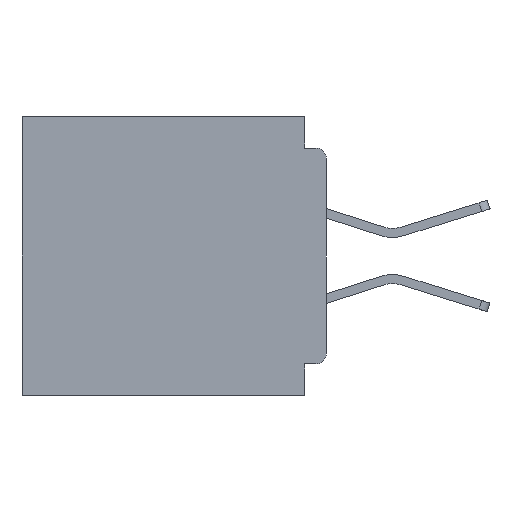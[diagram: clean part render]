
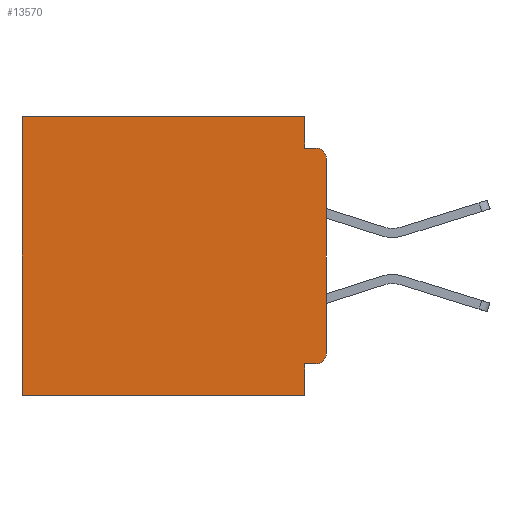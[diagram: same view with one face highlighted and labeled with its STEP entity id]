
A CAD part, left-side view. The second image highlights one B-rep face of the part: STEP entity #13570.
In plain terms, the highlighted planar face has unit normal (-1, 0, 0).
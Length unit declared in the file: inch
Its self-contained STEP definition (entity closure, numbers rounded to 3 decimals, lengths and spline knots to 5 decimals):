
#311 = EDGE_CURVE ( 'NONE', #14946, #16887, #39756, .T. ) ;
#653 = VECTOR ( 'NONE', #35557, 39.37008 ) ;
#1176 = VERTEX_POINT ( 'NONE', #3523 ) ;
#2168 = VERTEX_POINT ( 'NONE', #37568 ) ;
#3523 = CARTESIAN_POINT ( 'NONE',  ( 0.3, 0.031, -0.355 ) ) ;
#4334 = AXIS2_PLACEMENT_3D ( 'NONE', #11933, #9984, #10030 ) ;
#4850 = ORIENTED_EDGE ( 'NONE', *, *, #23393, .T. ) ;
#4950 = ORIENTED_EDGE ( 'NONE', *, *, #31621, .T. ) ;
#4956 = AXIS2_PLACEMENT_3D ( 'NONE', #25926, #29828, #6241 ) ;
#5565 = EDGE_CURVE ( 'NONE', #2168, #43491, #44742, .T. ) ;
#5735 = CARTESIAN_POINT ( 'NONE',  ( 0.3, 0.031, -0.045 ) ) ;
#6241 = DIRECTION ( 'NONE',  ( 0., 0., -1. ) ) ;
#8065 = CARTESIAN_POINT ( 'NONE',  ( 0.3, 0.437, -0.4 ) ) ;
#8159 = DIRECTION ( 'NONE',  ( 0., 0., -1. ) ) ;
#8387 = CARTESIAN_POINT ( 'NONE',  ( 0.3, 0., -0.34 ) ) ;
#9984 = DIRECTION ( 'NONE',  ( -1., 0., 0. ) ) ;
#10030 = DIRECTION ( 'NONE',  ( 0., 0., -1. ) ) ;
#10663 = ORIENTED_EDGE ( 'NONE', *, *, #46131, .F. ) ;
#10759 = DIRECTION ( 'NONE',  ( 0., 1., 0. ) ) ;
#11933 = CARTESIAN_POINT ( 'NONE',  ( 0.3, 0.015, -0.06 ) ) ;
#12539 = VECTOR ( 'NONE', #13088, 39.37008 ) ;
#13088 = DIRECTION ( 'NONE',  ( 0., 0., -1. ) ) ;
#13570 = ADVANCED_FACE ( 'NONE', ( #33282 ), #49184, .F. ) ;
#13924 = ORIENTED_EDGE ( 'NONE', *, *, #36365, .F. ) ;
#14374 = VERTEX_POINT ( 'NONE', #38635 ) ;
#14946 = VERTEX_POINT ( 'NONE', #18357 ) ;
#16887 = VERTEX_POINT ( 'NONE', #8387 ) ;
#17901 = LINE ( 'NONE', #8065, #653 ) ;
#18357 = CARTESIAN_POINT ( 'NONE',  ( 0.3, 0.015, -0.355 ) ) ;
#18718 = LINE ( 'NONE', #46426, #47393 ) ;
#19188 = LINE ( 'NONE', #28607, #38805 ) ;
#19637 = LINE ( 'NONE', #32131, #38030 ) ;
#20195 = LINE ( 'NONE', #35977, #46417 ) ;
#21438 = EDGE_CURVE ( 'NONE', #14946, #1176, #18718, .T. ) ;
#23393 = EDGE_CURVE ( 'NONE', #29288, #49319, #17901, .T. ) ;
#24069 = CARTESIAN_POINT ( 'NONE',  ( 0.3, 0.031, 0. ) ) ;
#24541 = VERTEX_POINT ( 'NONE', #5735 ) ;
#25926 = CARTESIAN_POINT ( 'NONE',  ( 0.3, 0., -0.4 ) ) ;
#26956 = ORIENTED_EDGE ( 'NONE', *, *, #5565, .T. ) ;
#27587 = CARTESIAN_POINT ( 'NONE',  ( 0.3, 0.437, -0.4 ) ) ;
#28607 = CARTESIAN_POINT ( 'NONE',  ( 0.3, 0., -0.045 ) ) ;
#29288 = VERTEX_POINT ( 'NONE', #43080 ) ;
#29828 = DIRECTION ( 'NONE',  ( 1., 0., 0. ) ) ;
#30958 = EDGE_CURVE ( 'NONE', #2168, #16887, #19637, .T. ) ;
#31077 = CARTESIAN_POINT ( 'NONE',  ( 0.3, 0.031, -0.4 ) ) ;
#31420 = EDGE_LOOP ( 'NONE', ( #39469, #26956, #32062, #37504, #4950, #4850, #13924, #10663, #32097, #32946 ) ) ;
#31621 = EDGE_CURVE ( 'NONE', #14374, #29288, #20195, .T. ) ;
#32062 = ORIENTED_EDGE ( 'NONE', *, *, #47541, .F. ) ;
#32097 = ORIENTED_EDGE ( 'NONE', *, *, #21438, .F. ) ;
#32131 = CARTESIAN_POINT ( 'NONE',  ( 0.3, 0., -0.4 ) ) ;
#32946 = ORIENTED_EDGE ( 'NONE', *, *, #311, .T. ) ;
#33282 = FACE_OUTER_BOUND ( 'NONE', #31420, .T. ) ;
#33768 = CARTESIAN_POINT ( 'NONE',  ( 0.3, 0.015, -0.045 ) ) ;
#34893 = DIRECTION ( 'NONE',  ( 0., 1., 0. ) ) ;
#35557 = DIRECTION ( 'NONE',  ( 0., 0., -1. ) ) ;
#35602 = VECTOR ( 'NONE', #8159, 39.37008 ) ;
#35977 = CARTESIAN_POINT ( 'NONE',  ( 0.3, 0., 0. ) ) ;
#36038 = DIRECTION ( 'NONE',  ( 0., 0., -1. ) ) ;
#36232 = VECTOR ( 'NONE', #10759, 39.37008 ) ;
#36365 = EDGE_CURVE ( 'NONE', #48609, #49319, #46570, .T. ) ;
#36580 = CARTESIAN_POINT ( 'NONE',  ( 0.3, 0.031, -0.4 ) ) ;
#36820 = LINE ( 'NONE', #24069, #35602 ) ;
#37504 = ORIENTED_EDGE ( 'NONE', *, *, #48725, .F. ) ;
#37568 = CARTESIAN_POINT ( 'NONE',  ( 0.3, 0., -0.06 ) ) ;
#38030 = VECTOR ( 'NONE', #36038, 39.37008 ) ;
#38235 = CARTESIAN_POINT ( 'NONE',  ( 0.3, 0., -0.4 ) ) ;
#38635 = CARTESIAN_POINT ( 'NONE',  ( 0.3, 0.031, 0. ) ) ;
#38805 = VECTOR ( 'NONE', #47972, 39.37008 ) ;
#39469 = ORIENTED_EDGE ( 'NONE', *, *, #30958, .F. ) ;
#39599 = DIRECTION ( 'NONE',  ( 0., 0., -1. ) ) ;
#39756 = CIRCLE ( 'NONE', #43944, 0.015 ) ;
#43040 = DIRECTION ( 'NONE',  ( -1., 0., 0. ) ) ;
#43080 = CARTESIAN_POINT ( 'NONE',  ( 0.3, 0.437, 0. ) ) ;
#43491 = VERTEX_POINT ( 'NONE', #33768 ) ;
#43818 = LINE ( 'NONE', #36580, #12539 ) ;
#43836 = DIRECTION ( 'NONE',  ( 0., 1., 0. ) ) ;
#43944 = AXIS2_PLACEMENT_3D ( 'NONE', #44061, #43040, #39599 ) ;
#44061 = CARTESIAN_POINT ( 'NONE',  ( 0.3, 0.015, -0.34 ) ) ;
#44742 = CIRCLE ( 'NONE', #4334, 0.015 ) ;
#46131 = EDGE_CURVE ( 'NONE', #1176, #48609, #43818, .T. ) ;
#46417 = VECTOR ( 'NONE', #43836, 39.37008 ) ;
#46426 = CARTESIAN_POINT ( 'NONE',  ( 0.3, 0., -0.355 ) ) ;
#46570 = LINE ( 'NONE', #38235, #36232 ) ;
#47393 = VECTOR ( 'NONE', #34893, 39.37008 ) ;
#47541 = EDGE_CURVE ( 'NONE', #24541, #43491, #19188, .T. ) ;
#47972 = DIRECTION ( 'NONE',  ( 0., -1., 0. ) ) ;
#48609 = VERTEX_POINT ( 'NONE', #31077 ) ;
#48725 = EDGE_CURVE ( 'NONE', #14374, #24541, #36820, .T. ) ;
#49184 = PLANE ( 'NONE',  #4956 ) ;
#49319 = VERTEX_POINT ( 'NONE', #27587 ) ;
